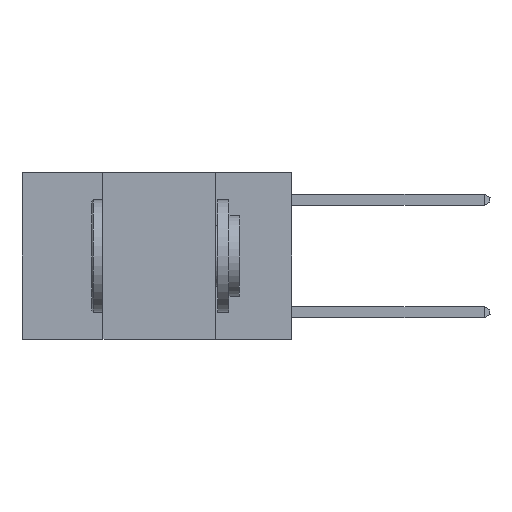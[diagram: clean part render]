
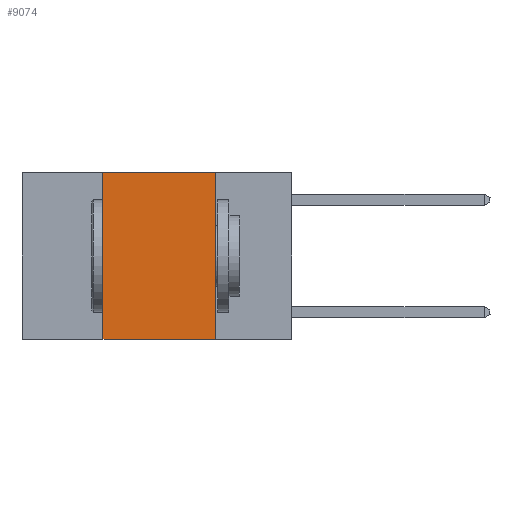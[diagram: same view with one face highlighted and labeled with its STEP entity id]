
A CAD part, left-side view. The second image highlights one B-rep face of the part: STEP entity #9074.
In plain terms, the highlighted planar face has unit normal (-1, 0, 0).
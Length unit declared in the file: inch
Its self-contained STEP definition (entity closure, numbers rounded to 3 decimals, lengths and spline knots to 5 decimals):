
#179 = VECTOR ( 'NONE', #12038, 39.37008 ) ;
#400 = DIRECTION ( 'NONE',  ( 0., 0., 1. ) ) ;
#1744 = VERTEX_POINT ( 'NONE', #4634 ) ;
#2642 = ORIENTED_EDGE ( 'NONE', *, *, #6099, .F. ) ;
#2767 = CARTESIAN_POINT ( 'NONE',  ( 0., 0.6, 0. ) ) ;
#3783 = CARTESIAN_POINT ( 'NONE',  ( 0., 0.6, 0. ) ) ;
#4169 = EDGE_CURVE ( 'NONE', #11755, #4233, #4811, .T. ) ;
#4233 = VERTEX_POINT ( 'NONE', #15624 ) ;
#4390 = DIRECTION ( 'NONE',  ( 1., 0., 0. ) ) ;
#4634 = CARTESIAN_POINT ( 'NONE',  ( 0., 0.42, 0. ) ) ;
#4643 = FACE_OUTER_BOUND ( 'NONE', #10622, .T. ) ;
#4811 = LINE ( 'NONE', #8958, #21208 ) ;
#4860 = CARTESIAN_POINT ( 'NONE',  ( 0., 0.42, 0. ) ) ;
#4873 = ORIENTED_EDGE ( 'NONE', *, *, #4169, .T. ) ;
#5837 = VERTEX_POINT ( 'NONE', #6535 ) ;
#6099 = EDGE_CURVE ( 'NONE', #5837, #4233, #25298, .T. ) ;
#6384 = ORIENTED_EDGE ( 'NONE', *, *, #15436, .F. ) ;
#6405 = PLANE ( 'NONE',  #14532 ) ;
#6535 = CARTESIAN_POINT ( 'NONE',  ( 0., 0.17, 0. ) ) ;
#6857 = CARTESIAN_POINT ( 'NONE',  ( 0., 0.17, 0. ) ) ;
#8958 = CARTESIAN_POINT ( 'NONE',  ( 0., 0.6, -0.37 ) ) ;
#9074 = ADVANCED_FACE ( 'NONE', ( #4643 ), #6405, .F. ) ;
#10622 = EDGE_LOOP ( 'NONE', ( #2642, #6384, #26219, #4873 ) ) ;
#11755 = VERTEX_POINT ( 'NONE', #14535 ) ;
#12038 = DIRECTION ( 'NONE',  ( 0., -1., 0. ) ) ;
#12302 = LINE ( 'NONE', #3783, #179 ) ;
#14532 = AXIS2_PLACEMENT_3D ( 'NONE', #2767, #4390, #18831 ) ;
#14535 = CARTESIAN_POINT ( 'NONE',  ( 0., 0.42, -0.37 ) ) ;
#15229 = DIRECTION ( 'NONE',  ( 0., -1., 0. ) ) ;
#15436 = EDGE_CURVE ( 'NONE', #1744, #5837, #12302, .T. ) ;
#15624 = CARTESIAN_POINT ( 'NONE',  ( 0., 0.17, -0.37 ) ) ;
#17843 = VECTOR ( 'NONE', #400, 39.37008 ) ;
#18831 = DIRECTION ( 'NONE',  ( 0., 0., -1. ) ) ;
#21009 = VECTOR ( 'NONE', #25960, 39.37008 ) ;
#21208 = VECTOR ( 'NONE', #15229, 39.37008 ) ;
#23316 = LINE ( 'NONE', #4860, #17843 ) ;
#25298 = LINE ( 'NONE', #6857, #21009 ) ;
#25462 = EDGE_CURVE ( 'NONE', #11755, #1744, #23316, .T. ) ;
#25960 = DIRECTION ( 'NONE',  ( 0., 0., -1. ) ) ;
#26219 = ORIENTED_EDGE ( 'NONE', *, *, #25462, .F. ) ;
